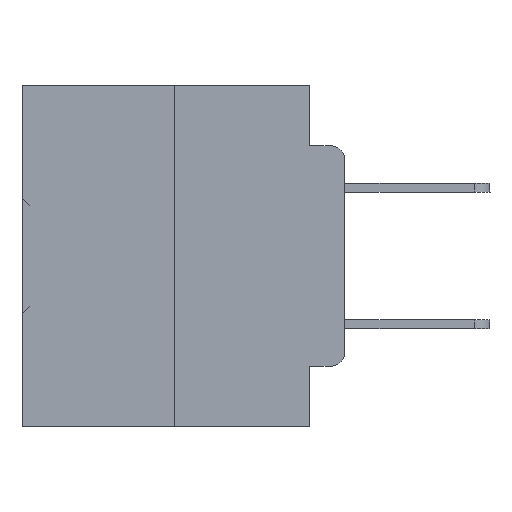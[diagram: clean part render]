
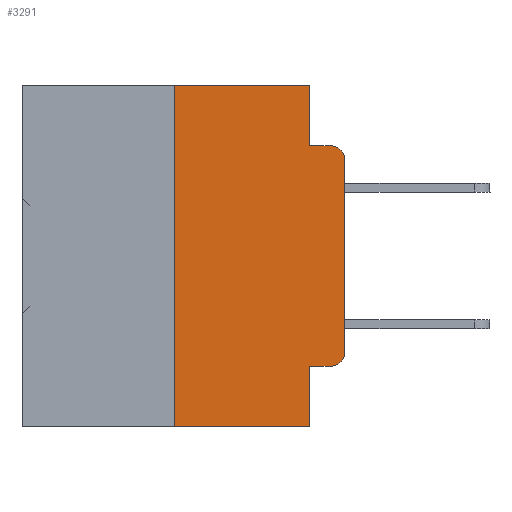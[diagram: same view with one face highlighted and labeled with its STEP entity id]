
A CAD part, left-side view. The second image highlights one B-rep face of the part: STEP entity #3291.
In plain terms, the highlighted planar face has unit normal (-1, 0, 0).
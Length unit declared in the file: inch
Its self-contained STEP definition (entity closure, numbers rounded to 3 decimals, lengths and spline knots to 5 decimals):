
#236 = CARTESIAN_POINT ( 'NONE',  ( 0., 0.473, -0.5 ) ) ;
#350 = DIRECTION ( 'NONE',  ( 0., 0., -1. ) ) ;
#1489 = VECTOR ( 'NONE', #7889, 39.37008 ) ;
#2343 = LINE ( 'NONE', #21434, #24384 ) ;
#2475 = LINE ( 'NONE', #37776, #1489 ) ;
#3291 = ADVANCED_FACE ( 'NONE', ( #19582 ), #7055, .F. ) ;
#3591 = CIRCLE ( 'NONE', #32820, 0.02 ) ;
#4612 = LINE ( 'NONE', #236, #12994 ) ;
#5912 = DIRECTION ( 'NONE',  ( 0., -1., 0. ) ) ;
#6369 = EDGE_CURVE ( 'NONE', #35446, #24302, #37016, .T. ) ;
#6704 = EDGE_LOOP ( 'NONE', ( #15707, #14368, #36415, #16174, #20955, #33813, #19579, #28108, #36438, #8526 ) ) ;
#7055 = PLANE ( 'NONE',  #14003 ) ;
#7184 = DIRECTION ( 'NONE',  ( 1., 0., 0. ) ) ;
#7239 = EDGE_CURVE ( 'NONE', #9611, #30767, #4612, .T. ) ;
#7595 = DIRECTION ( 'NONE',  ( 0., 0., -1. ) ) ;
#7889 = DIRECTION ( 'NONE',  ( 0., 0., 1. ) ) ;
#8526 = ORIENTED_EDGE ( 'NONE', *, *, #22088, .T. ) ;
#9473 = AXIS2_PLACEMENT_3D ( 'NONE', #25586, #37626, #7595 ) ;
#9611 = VERTEX_POINT ( 'NONE', #17630 ) ;
#9831 = VERTEX_POINT ( 'NONE', #20131 ) ;
#11115 = DIRECTION ( 'NONE',  ( 0., 0., -1. ) ) ;
#12101 = EDGE_CURVE ( 'NONE', #24986, #33233, #24331, .T. ) ;
#12558 = EDGE_CURVE ( 'NONE', #9611, #9831, #28558, .T. ) ;
#12586 = VECTOR ( 'NONE', #30900, 39.37008 ) ;
#12994 = VECTOR ( 'NONE', #5912, 39.37008 ) ;
#14003 = AXIS2_PLACEMENT_3D ( 'NONE', #25161, #7184, #33836 ) ;
#14368 = ORIENTED_EDGE ( 'NONE', *, *, #30101, .T. ) ;
#15707 = ORIENTED_EDGE ( 'NONE', *, *, #33331, .T. ) ;
#15883 = DIRECTION ( 'NONE',  ( 0., -1., 0. ) ) ;
#16174 = ORIENTED_EDGE ( 'NONE', *, *, #37642, .F. ) ;
#17630 = CARTESIAN_POINT ( 'NONE',  ( 0., 0.25, -0.5 ) ) ;
#17692 = CARTESIAN_POINT ( 'NONE',  ( 0., 0.02, -0.4115 ) ) ;
#19479 = VECTOR ( 'NONE', #350, 39.37008 ) ;
#19577 = CARTESIAN_POINT ( 'NONE',  ( 0., 0.051, -0.5 ) ) ;
#19579 = ORIENTED_EDGE ( 'NONE', *, *, #7239, .T. ) ;
#19582 = FACE_OUTER_BOUND ( 'NONE', #6704, .T. ) ;
#19797 = EDGE_CURVE ( 'NONE', #35446, #30767, #34506, .T. ) ;
#20131 = CARTESIAN_POINT ( 'NONE',  ( 0., 0.25, 0. ) ) ;
#20492 = VERTEX_POINT ( 'NONE', #24188 ) ;
#20955 = ORIENTED_EDGE ( 'NONE', *, *, #23384, .F. ) ;
#20994 = DIRECTION ( 'NONE',  ( 0., -1., 0. ) ) ;
#21434 = CARTESIAN_POINT ( 'NONE',  ( 0., 0.473, 0. ) ) ;
#22088 = EDGE_CURVE ( 'NONE', #24302, #37483, #22477, .T. ) ;
#22187 = CARTESIAN_POINT ( 'NONE',  ( 0., 0.02, -0.0885 ) ) ;
#22477 = CIRCLE ( 'NONE', #9473, 0.02 ) ;
#23384 = EDGE_CURVE ( 'NONE', #9831, #24829, #2343, .T. ) ;
#23873 = CARTESIAN_POINT ( 'NONE',  ( 0., 0.051, 0. ) ) ;
#24158 = LINE ( 'NONE', #38006, #26537 ) ;
#24188 = CARTESIAN_POINT ( 'NONE',  ( 0., 0., -0.1085 ) ) ;
#24302 = VERTEX_POINT ( 'NONE', #17692 ) ;
#24331 = LINE ( 'NONE', #36091, #34230 ) ;
#24384 = VECTOR ( 'NONE', #15883, 39.37008 ) ;
#24829 = VERTEX_POINT ( 'NONE', #23873 ) ;
#24986 = VERTEX_POINT ( 'NONE', #25051 ) ;
#25051 = CARTESIAN_POINT ( 'NONE',  ( 0., 0.051, -0.0885 ) ) ;
#25161 = CARTESIAN_POINT ( 'NONE',  ( 0., 0.473, 0. ) ) ;
#25586 = CARTESIAN_POINT ( 'NONE',  ( 0., 0.02, -0.3915 ) ) ;
#26537 = VECTOR ( 'NONE', #11115, 39.37008 ) ;
#27993 = CARTESIAN_POINT ( 'NONE',  ( 0., 0.051, -0.4115 ) ) ;
#28108 = ORIENTED_EDGE ( 'NONE', *, *, #19797, .F. ) ;
#28558 = LINE ( 'NONE', #30769, #12586 ) ;
#28567 = VECTOR ( 'NONE', #37289, 39.37008 ) ;
#30101 = EDGE_CURVE ( 'NONE', #20492, #33233, #3591, .T. ) ;
#30599 = DIRECTION ( 'NONE',  ( 0., 0., -1. ) ) ;
#30767 = VERTEX_POINT ( 'NONE', #19577 ) ;
#30769 = CARTESIAN_POINT ( 'NONE',  ( 0., 0.25, 0. ) ) ;
#30900 = DIRECTION ( 'NONE',  ( 0., 0., 1. ) ) ;
#31202 = CARTESIAN_POINT ( 'NONE',  ( 0., 0., -0.3915 ) ) ;
#32820 = AXIS2_PLACEMENT_3D ( 'NONE', #36771, #34043, #30599 ) ;
#33233 = VERTEX_POINT ( 'NONE', #22187 ) ;
#33271 = CARTESIAN_POINT ( 'NONE',  ( 0., 0.051, -0.4115 ) ) ;
#33310 = CARTESIAN_POINT ( 'NONE',  ( 0., 0.051, 0. ) ) ;
#33331 = EDGE_CURVE ( 'NONE', #37483, #20492, #2475, .T. ) ;
#33813 = ORIENTED_EDGE ( 'NONE', *, *, #12558, .F. ) ;
#33836 = DIRECTION ( 'NONE',  ( 0., 0., -1. ) ) ;
#34043 = DIRECTION ( 'NONE',  ( -1., 0., 0. ) ) ;
#34230 = VECTOR ( 'NONE', #20994, 39.37008 ) ;
#34506 = LINE ( 'NONE', #33310, #19479 ) ;
#35446 = VERTEX_POINT ( 'NONE', #33271 ) ;
#36091 = CARTESIAN_POINT ( 'NONE',  ( 0., 0.051, -0.0885 ) ) ;
#36415 = ORIENTED_EDGE ( 'NONE', *, *, #12101, .F. ) ;
#36438 = ORIENTED_EDGE ( 'NONE', *, *, #6369, .T. ) ;
#36771 = CARTESIAN_POINT ( 'NONE',  ( 0., 0.02, -0.1085 ) ) ;
#37016 = LINE ( 'NONE', #27993, #28567 ) ;
#37289 = DIRECTION ( 'NONE',  ( 0., -1., 0. ) ) ;
#37483 = VERTEX_POINT ( 'NONE', #31202 ) ;
#37626 = DIRECTION ( 'NONE',  ( -1., 0., 0. ) ) ;
#37642 = EDGE_CURVE ( 'NONE', #24829, #24986, #24158, .T. ) ;
#37776 = CARTESIAN_POINT ( 'NONE',  ( 0., 0., 0. ) ) ;
#38006 = CARTESIAN_POINT ( 'NONE',  ( 0., 0.051, 0. ) ) ;
